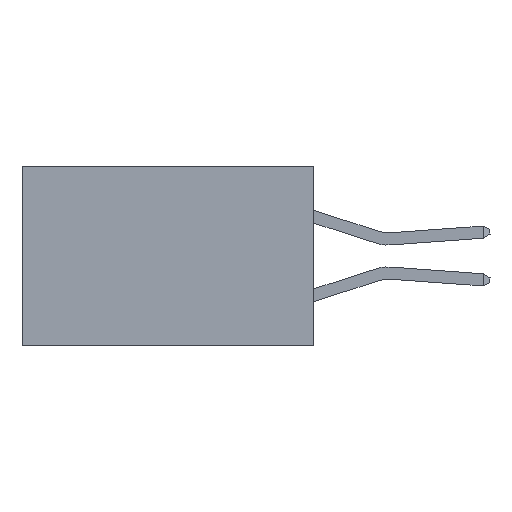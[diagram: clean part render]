
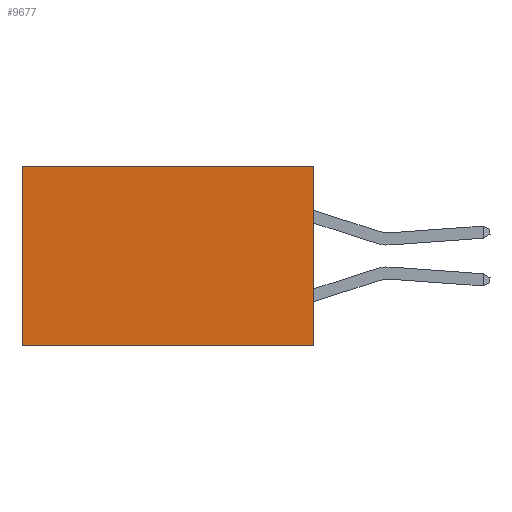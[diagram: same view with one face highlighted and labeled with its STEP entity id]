
A CAD part, left-side view. The second image highlights one B-rep face of the part: STEP entity #9677.
In plain terms, the highlighted planar face has unit normal (-1, 0, 0).
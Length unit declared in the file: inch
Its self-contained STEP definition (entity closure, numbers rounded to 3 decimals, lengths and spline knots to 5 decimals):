
#376 = DIRECTION ( 'NONE',  ( 0., 1., 0. ) ) ;
#1755 = PLANE ( 'NONE',  #21825 ) ;
#2351 = VERTEX_POINT ( 'NONE', #20673 ) ;
#4197 = CARTESIAN_POINT ( 'NONE',  ( 0.2875, 0., 0. ) ) ;
#5164 = ORIENTED_EDGE ( 'NONE', *, *, #20782, .F. ) ;
#5166 = VERTEX_POINT ( 'NONE', #21489 ) ;
#8564 = VECTOR ( 'NONE', #376, 39.37008 ) ;
#8808 = ORIENTED_EDGE ( 'NONE', *, *, #10832, .T. ) ;
#8928 = LINE ( 'NONE', #13825, #29348 ) ;
#9382 = DIRECTION ( 'NONE',  ( 0., 0., -1. ) ) ;
#9677 = ADVANCED_FACE ( 'NONE', ( #23688 ), #1755, .F. ) ;
#10590 = LINE ( 'NONE', #22852, #29423 ) ;
#10832 = EDGE_CURVE ( 'NONE', #29325, #24978, #21711, .T. ) ;
#11059 = EDGE_CURVE ( 'NONE', #24978, #2351, #8928, .T. ) ;
#13298 = ORIENTED_EDGE ( 'NONE', *, *, #24833, .F. ) ;
#13825 = CARTESIAN_POINT ( 'NONE',  ( 0.2875, 0.6, 0. ) ) ;
#13836 = CARTESIAN_POINT ( 'NONE',  ( 0.2875, 0., 0. ) ) ;
#16948 = DIRECTION ( 'NONE',  ( 0., 0., -1. ) ) ;
#17564 = CARTESIAN_POINT ( 'NONE',  ( 0.2875, 0.6, 0. ) ) ;
#18784 = ORIENTED_EDGE ( 'NONE', *, *, #11059, .T. ) ;
#19188 = EDGE_LOOP ( 'NONE', ( #18784, #5164, #13298, #8808 ) ) ;
#20673 = CARTESIAN_POINT ( 'NONE',  ( 0.2875, 0.6, -0.37 ) ) ;
#20782 = EDGE_CURVE ( 'NONE', #5166, #2351, #10590, .T. ) ;
#21018 = VECTOR ( 'NONE', #16948, 39.37008 ) ;
#21489 = CARTESIAN_POINT ( 'NONE',  ( 0.2875, 0., -0.37 ) ) ;
#21711 = LINE ( 'NONE', #30092, #8564 ) ;
#21825 = AXIS2_PLACEMENT_3D ( 'NONE', #4197, #24119, #9382 ) ;
#22852 = CARTESIAN_POINT ( 'NONE',  ( 0.2875, 0., -0.37 ) ) ;
#23688 = FACE_OUTER_BOUND ( 'NONE', #19188, .T. ) ;
#24119 = DIRECTION ( 'NONE',  ( 1., 0., 0. ) ) ;
#24833 = EDGE_CURVE ( 'NONE', #29325, #5166, #28289, .T. ) ;
#24978 = VERTEX_POINT ( 'NONE', #17564 ) ;
#25286 = DIRECTION ( 'NONE',  ( 0., 1., 0. ) ) ;
#28289 = LINE ( 'NONE', #31594, #21018 ) ;
#29325 = VERTEX_POINT ( 'NONE', #13836 ) ;
#29348 = VECTOR ( 'NONE', #30956, 39.37008 ) ;
#29423 = VECTOR ( 'NONE', #25286, 39.37008 ) ;
#30092 = CARTESIAN_POINT ( 'NONE',  ( 0.2875, 0., 0. ) ) ;
#30956 = DIRECTION ( 'NONE',  ( 0., 0., -1. ) ) ;
#31594 = CARTESIAN_POINT ( 'NONE',  ( 0.2875, 0., 0. ) ) ;
